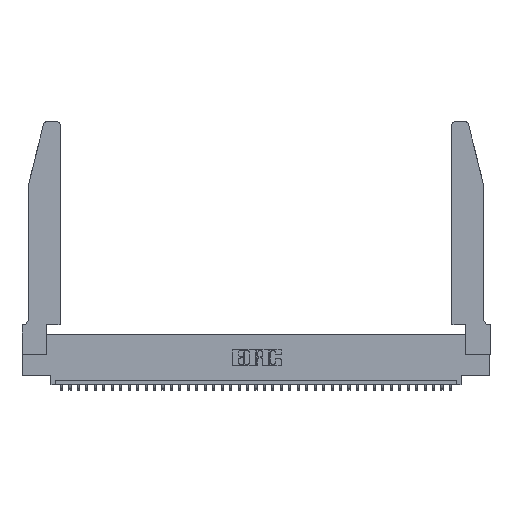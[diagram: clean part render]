
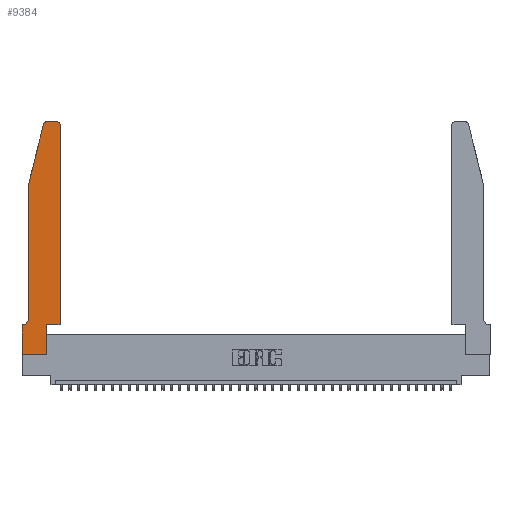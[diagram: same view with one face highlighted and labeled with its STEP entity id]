
A CAD part, top view. The second image highlights one B-rep face of the part: STEP entity #9384.
In plain terms, the highlighted planar face has unit normal (0, 0, 1).
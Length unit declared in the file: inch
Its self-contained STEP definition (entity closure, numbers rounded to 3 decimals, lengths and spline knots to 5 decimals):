
#399 = VERTEX_POINT ( 'NONE', #12098 ) ;
#624 = VERTEX_POINT ( 'NONE', #19226 ) ;
#711 = VERTEX_POINT ( 'NONE', #10868 ) ;
#816 = DIRECTION ( 'NONE',  ( 0., 0., 1. ) ) ;
#951 = DIRECTION ( 'NONE',  ( 1., 0., 0. ) ) ;
#1113 = VERTEX_POINT ( 'NONE', #29928 ) ;
#1216 = CARTESIAN_POINT ( 'NONE',  ( 0., 0.35, 0.37 ) ) ;
#1442 = DIRECTION ( 'NONE',  ( -1., 0., 0. ) ) ;
#1476 = VERTEX_POINT ( 'NONE', #16976 ) ;
#1512 = CARTESIAN_POINT ( 'NONE',  ( 0.2865, 0.35, 0.37 ) ) ;
#1809 = LINE ( 'NONE', #25243, #24825 ) ;
#2170 = VERTEX_POINT ( 'NONE', #11278 ) ;
#2357 = ORIENTED_EDGE ( 'NONE', *, *, #27642, .T. ) ;
#2455 = CARTESIAN_POINT ( 'NONE',  ( 0.4505, 0.35, 0.37 ) ) ;
#2562 = AXIS2_PLACEMENT_3D ( 'NONE', #13158, #37735, #1442 ) ;
#2757 = CARTESIAN_POINT ( 'NONE',  ( 0.0755, 0.35, 0.37 ) ) ;
#3077 = EDGE_CURVE ( 'NONE', #11219, #9958, #33127, .T. ) ;
#3081 = ORIENTED_EDGE ( 'NONE', *, *, #21158, .T. ) ;
#3407 = VERTEX_POINT ( 'NONE', #16815 ) ;
#3521 = ORIENTED_EDGE ( 'NONE', *, *, #8116, .T. ) ;
#3978 = LINE ( 'NONE', #22311, #12561 ) ;
#4152 = CARTESIAN_POINT ( 'NONE',  ( 0.0755, 2., 0.37 ) ) ;
#4350 = DIRECTION ( 'NONE',  ( -1., 0., 0. ) ) ;
#5773 = LINE ( 'NONE', #19689, #21160 ) ;
#6965 = ORIENTED_EDGE ( 'NONE', *, *, #18100, .T. ) ;
#7400 = ORIENTED_EDGE ( 'NONE', *, *, #36394, .T. ) ;
#7558 = DIRECTION ( 'NONE',  ( -0.239, -0.971, 0. ) ) ;
#8116 = EDGE_CURVE ( 'NONE', #624, #1113, #5773, .T. ) ;
#8333 = ORIENTED_EDGE ( 'NONE', *, *, #24813, .T. ) ;
#8646 = LINE ( 'NONE', #9948, #11496 ) ;
#9384 = ADVANCED_FACE ( 'NONE', ( #35861 ), #27035, .T. ) ;
#9853 = CARTESIAN_POINT ( 'NONE',  ( 0.0755, 0.42, 0.37 ) ) ;
#9864 = DIRECTION ( 'NONE',  ( 0., -1., 0. ) ) ;
#9948 = CARTESIAN_POINT ( 'NONE',  ( 0., 0., 0.37 ) ) ;
#9958 = VERTEX_POINT ( 'NONE', #15753 ) ;
#10534 = CIRCLE ( 'NONE', #36628, 0.03 ) ;
#10868 = CARTESIAN_POINT ( 'NONE',  ( 0.2865, 0.35, 0.37 ) ) ;
#11219 = VERTEX_POINT ( 'NONE', #11554 ) ;
#11278 = CARTESIAN_POINT ( 'NONE',  ( 0.4205, 2.75, 0.37 ) ) ;
#11496 = VECTOR ( 'NONE', #19266, 39.37008 ) ;
#11554 = CARTESIAN_POINT ( 'NONE',  ( 0.0055, 0.35, 0.37 ) ) ;
#12065 = DIRECTION ( 'NONE',  ( -1., 0., 0. ) ) ;
#12098 = CARTESIAN_POINT ( 'NONE',  ( 0.2865, 0., 0.37 ) ) ;
#12561 = VECTOR ( 'NONE', #28449, 39.37008 ) ;
#12867 = ORIENTED_EDGE ( 'NONE', *, *, #16602, .T. ) ;
#13158 = CARTESIAN_POINT ( 'NONE',  ( 0.0055, 0.42, 0.37 ) ) ;
#13533 = EDGE_LOOP ( 'NONE', ( #3081, #12867, #3521, #35990, #7400, #23282, #22554, #2357, #8333, #29992, #6965, #35340 ) ) ;
#13798 = DIRECTION ( 'NONE',  ( 0., 1., 0. ) ) ;
#14857 = VERTEX_POINT ( 'NONE', #16875 ) ;
#15465 = LINE ( 'NONE', #27816, #27048 ) ;
#15541 = VECTOR ( 'NONE', #29936, 39.37008 ) ;
#15753 = CARTESIAN_POINT ( 'NONE',  ( 0., 0.35, 0.37 ) ) ;
#16602 = EDGE_CURVE ( 'NONE', #3407, #624, #10534, .T. ) ;
#16815 = CARTESIAN_POINT ( 'NONE',  ( 0.284, 2.75, 0.37 ) ) ;
#16875 = CARTESIAN_POINT ( 'NONE',  ( 0., 0., 0.37 ) ) ;
#16976 = CARTESIAN_POINT ( 'NONE',  ( 0.4505, 2.72, 0.37 ) ) ;
#17623 = EDGE_CURVE ( 'NONE', #1113, #17932, #39272, .T. ) ;
#17932 = VERTEX_POINT ( 'NONE', #9853 ) ;
#18100 = EDGE_CURVE ( 'NONE', #29522, #1476, #1809, .T. ) ;
#18184 = VECTOR ( 'NONE', #9864, 39.37008 ) ;
#19226 = CARTESIAN_POINT ( 'NONE',  ( 0.25487, 2.72718, 0.37 ) ) ;
#19266 = DIRECTION ( 'NONE',  ( 0., -1., 0. ) ) ;
#19689 = CARTESIAN_POINT ( 'NONE',  ( 0.0755, 2., 0.37 ) ) ;
#20644 = AXIS2_PLACEMENT_3D ( 'NONE', #1216, #32505, #26560 ) ;
#21158 = EDGE_CURVE ( 'NONE', #2170, #3407, #15465, .T. ) ;
#21160 = VECTOR ( 'NONE', #7558, 39.37008 ) ;
#21774 = LINE ( 'NONE', #1512, #26052 ) ;
#22311 = CARTESIAN_POINT ( 'NONE',  ( 0.4505, 0.35, 0.37 ) ) ;
#22554 = ORIENTED_EDGE ( 'NONE', *, *, #30204, .T. ) ;
#23282 = ORIENTED_EDGE ( 'NONE', *, *, #3077, .T. ) ;
#23654 = DIRECTION ( 'NONE',  ( 1., 0., 0. ) ) ;
#24813 = EDGE_CURVE ( 'NONE', #399, #711, #21774, .T. ) ;
#24825 = VECTOR ( 'NONE', #37623, 39.37008 ) ;
#25243 = CARTESIAN_POINT ( 'NONE',  ( 0.4505, 0.35, 0.37 ) ) ;
#26052 = VECTOR ( 'NONE', #13798, 39.37008 ) ;
#26395 = CIRCLE ( 'NONE', #2562, 0.07 ) ;
#26560 = DIRECTION ( 'NONE',  ( 1., 0., 0. ) ) ;
#27035 = PLANE ( 'NONE',  #20644 ) ;
#27048 = VECTOR ( 'NONE', #4350, 39.37008 ) ;
#27642 = EDGE_CURVE ( 'NONE', #14857, #399, #39578, .T. ) ;
#27816 = CARTESIAN_POINT ( 'NONE',  ( 0.2605, 2.75, 0.37 ) ) ;
#28237 = AXIS2_PLACEMENT_3D ( 'NONE', #39269, #35829, #23654 ) ;
#28449 = DIRECTION ( 'NONE',  ( 1., 0., 0. ) ) ;
#29522 = VERTEX_POINT ( 'NONE', #2455 ) ;
#29928 = CARTESIAN_POINT ( 'NONE',  ( 0.0755, 2., 0.37 ) ) ;
#29936 = DIRECTION ( 'NONE',  ( 1., 0., 0. ) ) ;
#29992 = ORIENTED_EDGE ( 'NONE', *, *, #33793, .T. ) ;
#30204 = EDGE_CURVE ( 'NONE', #9958, #14857, #8646, .T. ) ;
#30657 = CIRCLE ( 'NONE', #28237, 0.03 ) ;
#32161 = VECTOR ( 'NONE', #12065, 39.37008 ) ;
#32505 = DIRECTION ( 'NONE',  ( 0., 0., 1. ) ) ;
#33127 = LINE ( 'NONE', #2757, #32161 ) ;
#33793 = EDGE_CURVE ( 'NONE', #711, #29522, #3978, .T. ) ;
#34607 = CARTESIAN_POINT ( 'NONE',  ( 0.284, 2.72, 0.37 ) ) ;
#35340 = ORIENTED_EDGE ( 'NONE', *, *, #36040, .T. ) ;
#35441 = CARTESIAN_POINT ( 'NONE',  ( 0., 0., 0.37 ) ) ;
#35829 = DIRECTION ( 'NONE',  ( 0., 0., 1. ) ) ;
#35861 = FACE_OUTER_BOUND ( 'NONE', #13533, .T. ) ;
#35990 = ORIENTED_EDGE ( 'NONE', *, *, #17623, .T. ) ;
#36040 = EDGE_CURVE ( 'NONE', #1476, #2170, #30657, .T. ) ;
#36394 = EDGE_CURVE ( 'NONE', #17932, #11219, #26395, .T. ) ;
#36628 = AXIS2_PLACEMENT_3D ( 'NONE', #34607, #816, #951 ) ;
#37623 = DIRECTION ( 'NONE',  ( 0., 1., 0. ) ) ;
#37735 = DIRECTION ( 'NONE',  ( 0., 0., -1. ) ) ;
#39269 = CARTESIAN_POINT ( 'NONE',  ( 0.4205, 2.72, 0.37 ) ) ;
#39272 = LINE ( 'NONE', #4152, #18184 ) ;
#39578 = LINE ( 'NONE', #35441, #15541 ) ;
